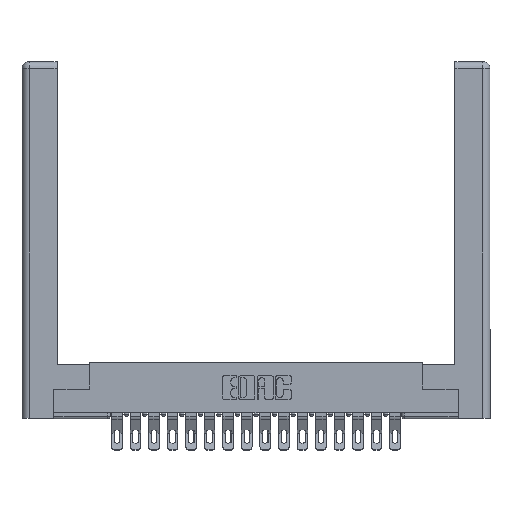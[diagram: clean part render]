
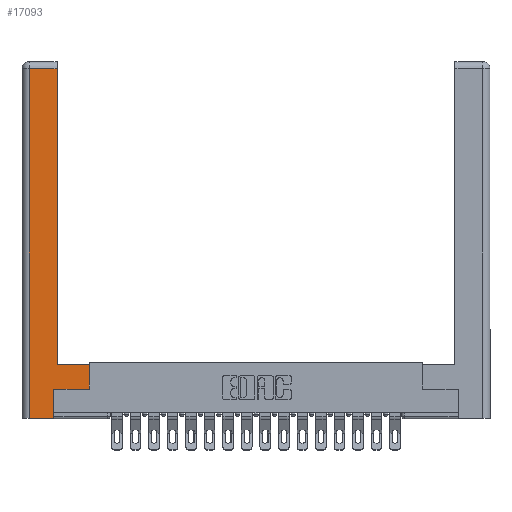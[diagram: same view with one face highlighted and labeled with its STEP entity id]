
A CAD part, top view. The second image highlights one B-rep face of the part: STEP entity #17093.
In plain terms, the highlighted planar face has unit normal (0, 0, 1).
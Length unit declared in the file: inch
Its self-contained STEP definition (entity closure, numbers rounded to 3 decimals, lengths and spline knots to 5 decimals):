
#180 = DIRECTION ( 'NONE',  ( 0., -1., 0. ) ) ;
#627 = CARTESIAN_POINT ( 'NONE',  ( 0.565, 0.45, 0. ) ) ;
#679 = VERTEX_POINT ( 'NONE', #7764 ) ;
#796 = VECTOR ( 'NONE', #17109, 39.37008 ) ;
#852 = VERTEX_POINT ( 'NONE', #8587 ) ;
#922 = CARTESIAN_POINT ( 'NONE',  ( 0.0615, 2.94, 0. ) ) ;
#1024 = DIRECTION ( 'NONE',  ( 1., 0., 0. ) ) ;
#1675 = ORIENTED_EDGE ( 'NONE', *, *, #5564, .T. ) ;
#2322 = CARTESIAN_POINT ( 'NONE',  ( 0.295, 2.94, 0. ) ) ;
#2452 = PLANE ( 'NONE',  #17454 ) ;
#2763 = LINE ( 'NONE', #10902, #8649 ) ;
#3132 = ORIENTED_EDGE ( 'NONE', *, *, #3940, .T. ) ;
#3339 = DIRECTION ( 'NONE',  ( -1., 0., 0. ) ) ;
#3478 = VECTOR ( 'NONE', #180, 39.37008 ) ;
#3512 = ORIENTED_EDGE ( 'NONE', *, *, #8627, .T. ) ;
#3560 = CARTESIAN_POINT ( 'NONE',  ( 0.265, 0.245, 0. ) ) ;
#3703 = FACE_OUTER_BOUND ( 'NONE', #16923, .T. ) ;
#3817 = VERTEX_POINT ( 'NONE', #3560 ) ;
#3913 = EDGE_CURVE ( 'NONE', #3817, #852, #7419, .T. ) ;
#3940 = EDGE_CURVE ( 'NONE', #20243, #679, #10942, .T. ) ;
#4851 = ORIENTED_EDGE ( 'NONE', *, *, #13590, .T. ) ;
#5321 = LINE ( 'NONE', #7106, #12055 ) ;
#5424 = ORIENTED_EDGE ( 'NONE', *, *, #8715, .T. ) ;
#5550 = VECTOR ( 'NONE', #17364, 39.37008 ) ;
#5564 = EDGE_CURVE ( 'NONE', #9850, #20243, #7402, .T. ) ;
#5821 = VECTOR ( 'NONE', #13653, 39.37008 ) ;
#6322 = LINE ( 'NONE', #12679, #11532 ) ;
#6351 = VERTEX_POINT ( 'NONE', #10450 ) ;
#6371 = CARTESIAN_POINT ( 'NONE',  ( 0.0615, 2.94, 0. ) ) ;
#7106 = CARTESIAN_POINT ( 'NONE',  ( 0.265, 0., 0. ) ) ;
#7402 = LINE ( 'NONE', #922, #5821 ) ;
#7419 = LINE ( 'NONE', #10740, #796 ) ;
#7764 = CARTESIAN_POINT ( 'NONE',  ( 0.0615, 0., 0. ) ) ;
#7997 = ORIENTED_EDGE ( 'NONE', *, *, #3913, .T. ) ;
#8587 = CARTESIAN_POINT ( 'NONE',  ( 0.565, 0.245, 0. ) ) ;
#8627 = EDGE_CURVE ( 'NONE', #852, #18716, #2763, .T. ) ;
#8649 = VECTOR ( 'NONE', #15494, 39.37008 ) ;
#8715 = EDGE_CURVE ( 'NONE', #6351, #3817, #20599, .T. ) ;
#8727 = EDGE_CURVE ( 'NONE', #18716, #14559, #6322, .T. ) ;
#9850 = VERTEX_POINT ( 'NONE', #2322 ) ;
#10450 = CARTESIAN_POINT ( 'NONE',  ( 0.265, 0., 0. ) ) ;
#10740 = CARTESIAN_POINT ( 'NONE',  ( 0.565, 0.245, 0. ) ) ;
#10877 = ORIENTED_EDGE ( 'NONE', *, *, #8727, .T. ) ;
#10902 = CARTESIAN_POINT ( 'NONE',  ( 0.565, 0.45, 0. ) ) ;
#10942 = LINE ( 'NONE', #14491, #3478 ) ;
#11359 = EDGE_CURVE ( 'NONE', #14559, #9850, #16952, .T. ) ;
#11532 = VECTOR ( 'NONE', #3339, 39.37008 ) ;
#12055 = VECTOR ( 'NONE', #1024, 39.37008 ) ;
#12679 = CARTESIAN_POINT ( 'NONE',  ( 0.295, 0.45, 0. ) ) ;
#13410 = CARTESIAN_POINT ( 'NONE',  ( 0., 0., 0. ) ) ;
#13590 = EDGE_CURVE ( 'NONE', #679, #6351, #5321, .T. ) ;
#13653 = DIRECTION ( 'NONE',  ( -1., 0., 0. ) ) ;
#14008 = CARTESIAN_POINT ( 'NONE',  ( 0.295, 0.45, 0. ) ) ;
#14241 = ORIENTED_EDGE ( 'NONE', *, *, #11359, .T. ) ;
#14491 = CARTESIAN_POINT ( 'NONE',  ( 0.0615, 0., 0. ) ) ;
#14559 = VERTEX_POINT ( 'NONE', #14008 ) ;
#14973 = VECTOR ( 'NONE', #17052, 39.37008 ) ;
#15073 = DIRECTION ( 'NONE',  ( 0., 0., -1. ) ) ;
#15494 = DIRECTION ( 'NONE',  ( 0., 1., 0. ) ) ;
#15688 = CARTESIAN_POINT ( 'NONE',  ( 0.295, 3., 0. ) ) ;
#16642 = DIRECTION ( 'NONE',  ( -1., 0., 0. ) ) ;
#16923 = EDGE_LOOP ( 'NONE', ( #14241, #1675, #3132, #4851, #5424, #7997, #3512, #10877 ) ) ;
#16952 = LINE ( 'NONE', #15688, #14973 ) ;
#17052 = DIRECTION ( 'NONE',  ( 0., 1., 0. ) ) ;
#17093 = ADVANCED_FACE ( 'NONE', ( #3703 ), #2452, .F. ) ;
#17109 = DIRECTION ( 'NONE',  ( 1., 0., 0. ) ) ;
#17364 = DIRECTION ( 'NONE',  ( 0., 1., 0. ) ) ;
#17454 = AXIS2_PLACEMENT_3D ( 'NONE', #13410, #15073, #16642 ) ;
#18716 = VERTEX_POINT ( 'NONE', #627 ) ;
#18937 = CARTESIAN_POINT ( 'NONE',  ( 0.265, 0.245, 0. ) ) ;
#20243 = VERTEX_POINT ( 'NONE', #6371 ) ;
#20599 = LINE ( 'NONE', #18937, #5550 ) ;
